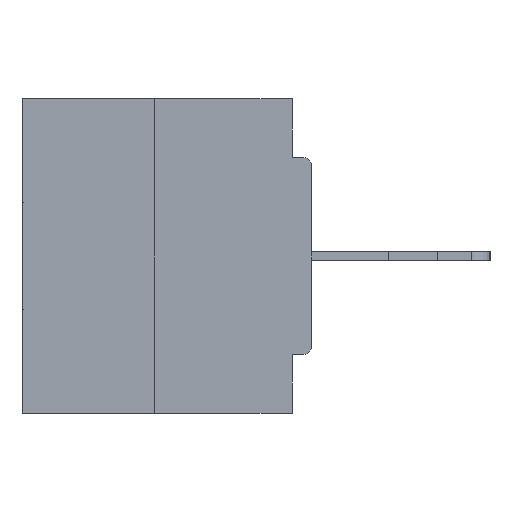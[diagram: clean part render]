
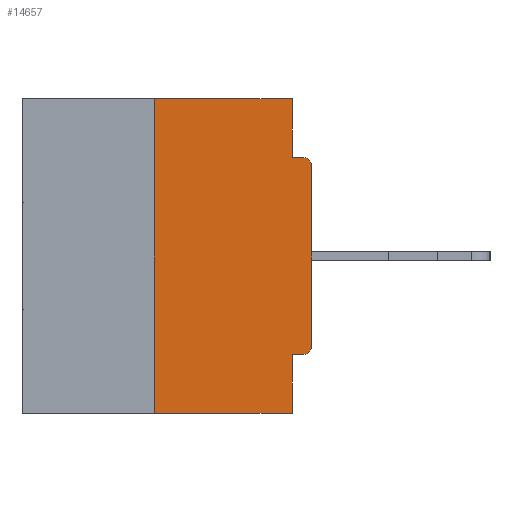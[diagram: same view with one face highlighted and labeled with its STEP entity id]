
A CAD part, left-side view. The second image highlights one B-rep face of the part: STEP entity #14657.
In plain terms, the highlighted planar face has unit normal (-1, 0, 0).
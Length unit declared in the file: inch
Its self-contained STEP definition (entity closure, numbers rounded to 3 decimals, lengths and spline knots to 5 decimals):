
#461 = EDGE_CURVE ( 'NONE', #33641, #1636, #25196, .T. ) ;
#587 = DIRECTION ( 'NONE',  ( 0., 0., -1. ) ) ;
#1361 = DIRECTION ( 'NONE',  ( 0., -1., 0. ) ) ;
#1636 = VERTEX_POINT ( 'NONE', #24985 ) ;
#1764 = DIRECTION ( 'NONE',  ( 0., 1., 0. ) ) ;
#2207 = VECTOR ( 'NONE', #14574, 39.37008 ) ;
#3066 = VECTOR ( 'NONE', #21080, 39.37008 ) ;
#3169 = PLANE ( 'NONE',  #16566 ) ;
#3279 = CARTESIAN_POINT ( 'NONE',  ( 0., 0.46, 0. ) ) ;
#3337 = VERTEX_POINT ( 'NONE', #19070 ) ;
#3394 = VECTOR ( 'NONE', #33818, 39.37008 ) ;
#4204 = EDGE_LOOP ( 'NONE', ( #28131, #22691, #4235, #26075, #7518, #21457, #30205, #25678, #20266, #29820 ) ) ;
#4235 = ORIENTED_EDGE ( 'NONE', *, *, #6447, .T. ) ;
#5543 = CARTESIAN_POINT ( 'NONE',  ( 0., 0.031, -0.0935 ) ) ;
#5788 = DIRECTION ( 'NONE',  ( 0., 0., -1. ) ) ;
#6144 = CARTESIAN_POINT ( 'NONE',  ( 0., 0.25, -0.5 ) ) ;
#6447 = EDGE_CURVE ( 'NONE', #33641, #3337, #31888, .T. ) ;
#6787 = EDGE_CURVE ( 'NONE', #9618, #30322, #13264, .T. ) ;
#7131 = VECTOR ( 'NONE', #29583, 39.37008 ) ;
#7518 = ORIENTED_EDGE ( 'NONE', *, *, #13159, .F. ) ;
#7589 = CARTESIAN_POINT ( 'NONE',  ( 0., 0.015, -0.0935 ) ) ;
#8088 = LINE ( 'NONE', #3279, #28328 ) ;
#9618 = VERTEX_POINT ( 'NONE', #15849 ) ;
#10121 = CARTESIAN_POINT ( 'NONE',  ( 0., 0., -0.1085 ) ) ;
#11072 = EDGE_CURVE ( 'NONE', #30322, #26808, #20219, .T. ) ;
#13159 = EDGE_CURVE ( 'NONE', #15327, #23235, #23351, .T. ) ;
#13264 = LINE ( 'NONE', #30324, #7131 ) ;
#13785 = CARTESIAN_POINT ( 'NONE',  ( 0., 0.031, -0.4065 ) ) ;
#13911 = VECTOR ( 'NONE', #1361, 39.37008 ) ;
#13934 = CIRCLE ( 'NONE', #31636, 0.015 ) ;
#14363 = CARTESIAN_POINT ( 'NONE',  ( 0., 0.015, -0.1085 ) ) ;
#14396 = CARTESIAN_POINT ( 'NONE',  ( 0., 0., -0.0935 ) ) ;
#14574 = DIRECTION ( 'NONE',  ( 0., 0., -1. ) ) ;
#14657 = ADVANCED_FACE ( 'NONE', ( #29170 ), #3169, .F. ) ;
#14691 = EDGE_CURVE ( 'NONE', #1636, #32730, #8088, .T. ) ;
#15327 = VERTEX_POINT ( 'NONE', #32473 ) ;
#15849 = CARTESIAN_POINT ( 'NONE',  ( 0., 0., -0.3915 ) ) ;
#16119 = LINE ( 'NONE', #25120, #2207 ) ;
#16274 = DIRECTION ( 'NONE',  ( -1., 0., 0. ) ) ;
#16509 = CARTESIAN_POINT ( 'NONE',  ( 0., 0.46, -0.5 ) ) ;
#16566 = AXIS2_PLACEMENT_3D ( 'NONE', #29427, #21482, #5788 ) ;
#17018 = DIRECTION ( 'NONE',  ( 0., 0., -1. ) ) ;
#17458 = CARTESIAN_POINT ( 'NONE',  ( 0., 0., -0.4065 ) ) ;
#19070 = CARTESIAN_POINT ( 'NONE',  ( 0., 0.031, -0.5 ) ) ;
#19791 = EDGE_CURVE ( 'NONE', #21859, #26808, #28837, .T. ) ;
#19880 = LINE ( 'NONE', #20320, #33938 ) ;
#20219 = CIRCLE ( 'NONE', #29741, 0.015 ) ;
#20266 = ORIENTED_EDGE ( 'NONE', *, *, #19791, .F. ) ;
#20320 = CARTESIAN_POINT ( 'NONE',  ( 0., 0.031, -0.5 ) ) ;
#20627 = CARTESIAN_POINT ( 'NONE',  ( 0., 0.25, 0. ) ) ;
#21080 = DIRECTION ( 'NONE',  ( 0., -1., 0. ) ) ;
#21457 = ORIENTED_EDGE ( 'NONE', *, *, #32363, .T. ) ;
#21482 = DIRECTION ( 'NONE',  ( 1., 0., 0. ) ) ;
#21859 = VERTEX_POINT ( 'NONE', #5543 ) ;
#22292 = EDGE_CURVE ( 'NONE', #23235, #3337, #19880, .T. ) ;
#22691 = ORIENTED_EDGE ( 'NONE', *, *, #461, .F. ) ;
#23235 = VERTEX_POINT ( 'NONE', #13785 ) ;
#23351 = LINE ( 'NONE', #17458, #29611 ) ;
#24985 = CARTESIAN_POINT ( 'NONE',  ( 0., 0.25, 0. ) ) ;
#25120 = CARTESIAN_POINT ( 'NONE',  ( 0., 0.031, 0. ) ) ;
#25196 = LINE ( 'NONE', #20627, #3394 ) ;
#25678 = ORIENTED_EDGE ( 'NONE', *, *, #11072, .T. ) ;
#26075 = ORIENTED_EDGE ( 'NONE', *, *, #22292, .F. ) ;
#26808 = VERTEX_POINT ( 'NONE', #7589 ) ;
#28131 = ORIENTED_EDGE ( 'NONE', *, *, #14691, .F. ) ;
#28328 = VECTOR ( 'NONE', #32143, 39.37008 ) ;
#28837 = LINE ( 'NONE', #14396, #13911 ) ;
#29170 = FACE_OUTER_BOUND ( 'NONE', #4204, .T. ) ;
#29427 = CARTESIAN_POINT ( 'NONE',  ( 0., 0.46, 0. ) ) ;
#29583 = DIRECTION ( 'NONE',  ( 0., 0., 1. ) ) ;
#29611 = VECTOR ( 'NONE', #1764, 39.37008 ) ;
#29741 = AXIS2_PLACEMENT_3D ( 'NONE', #14363, #32867, #17018 ) ;
#29820 = ORIENTED_EDGE ( 'NONE', *, *, #30155, .F. ) ;
#30155 = EDGE_CURVE ( 'NONE', #32730, #21859, #16119, .T. ) ;
#30205 = ORIENTED_EDGE ( 'NONE', *, *, #6787, .T. ) ;
#30322 = VERTEX_POINT ( 'NONE', #10121 ) ;
#30324 = CARTESIAN_POINT ( 'NONE',  ( 0., 0., 0. ) ) ;
#31545 = CARTESIAN_POINT ( 'NONE',  ( 0., 0.031, 0. ) ) ;
#31636 = AXIS2_PLACEMENT_3D ( 'NONE', #32112, #16274, #587 ) ;
#31888 = LINE ( 'NONE', #16509, #3066 ) ;
#32112 = CARTESIAN_POINT ( 'NONE',  ( 0., 0.015, -0.3915 ) ) ;
#32143 = DIRECTION ( 'NONE',  ( 0., -1., 0. ) ) ;
#32363 = EDGE_CURVE ( 'NONE', #15327, #9618, #13934, .T. ) ;
#32473 = CARTESIAN_POINT ( 'NONE',  ( 0., 0.015, -0.4065 ) ) ;
#32730 = VERTEX_POINT ( 'NONE', #31545 ) ;
#32867 = DIRECTION ( 'NONE',  ( -1., 0., 0. ) ) ;
#33633 = DIRECTION ( 'NONE',  ( 0., 0., -1. ) ) ;
#33641 = VERTEX_POINT ( 'NONE', #6144 ) ;
#33818 = DIRECTION ( 'NONE',  ( 0., 0., 1. ) ) ;
#33938 = VECTOR ( 'NONE', #33633, 39.37008 ) ;
